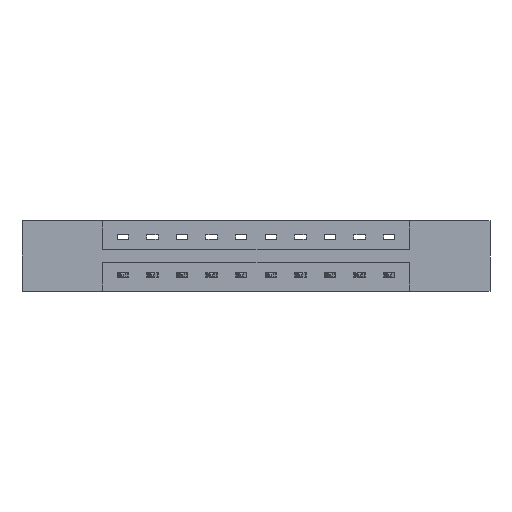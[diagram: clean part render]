
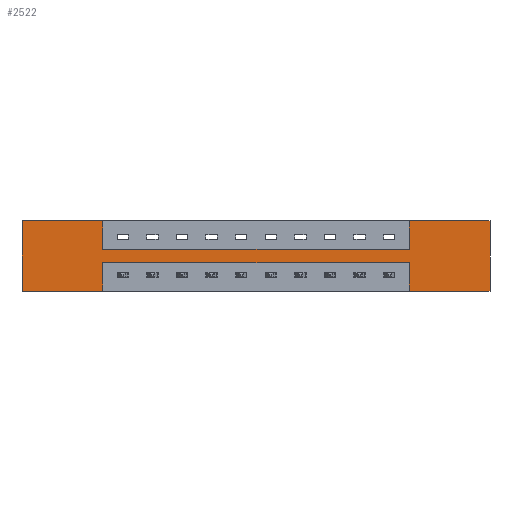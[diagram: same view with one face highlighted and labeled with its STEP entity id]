
A CAD part, front view. The second image highlights one B-rep face of the part: STEP entity #2522.
In plain terms, the highlighted planar face has unit normal (0, -1, 0).
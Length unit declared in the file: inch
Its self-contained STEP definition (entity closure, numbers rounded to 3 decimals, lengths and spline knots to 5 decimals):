
#37 = EDGE_LOOP ( 'NONE', ( #4826, #7178, #9392, #11586, #9649, #265, #9899, #571, #3261, #5677, #7989, #10137 ) ) ;
#176 = LINE ( 'NONE', #4265, #7356 ) ;
#265 = ORIENTED_EDGE ( 'NONE', *, *, #9397, .F. ) ;
#283 = CARTESIAN_POINT ( 'NONE',  ( 2.466, 0., -0.37 ) ) ;
#300 = DIRECTION ( 'NONE',  ( 1., 0., 0. ) ) ;
#311 = VECTOR ( 'NONE', #3619, 39.37008 ) ;
#571 = ORIENTED_EDGE ( 'NONE', *, *, #2666, .F. ) ;
#597 = VECTOR ( 'NONE', #9784, 39.37008 ) ;
#627 = VERTEX_POINT ( 'NONE', #11444 ) ;
#863 = DIRECTION ( 'NONE',  ( 0., -1., 0. ) ) ;
#895 = CARTESIAN_POINT ( 'NONE',  ( 2.041, 0., -0.15 ) ) ;
#914 = CARTESIAN_POINT ( 'NONE',  ( 0., 0., -0.37 ) ) ;
#1224 = VERTEX_POINT ( 'NONE', #1527 ) ;
#1290 = PLANE ( 'NONE',  #4752 ) ;
#1486 = VERTEX_POINT ( 'NONE', #4893 ) ;
#1527 = CARTESIAN_POINT ( 'NONE',  ( 2.466, 0., 0. ) ) ;
#1689 = EDGE_CURVE ( 'NONE', #1224, #8025, #7333, .T. ) ;
#1720 = CARTESIAN_POINT ( 'NONE',  ( 2.041, 0., -0.37 ) ) ;
#1885 = LINE ( 'NONE', #5284, #8769 ) ;
#1949 = EDGE_CURVE ( 'NONE', #8025, #1486, #5438, .T. ) ;
#2281 = CARTESIAN_POINT ( 'NONE',  ( 2.466, 0., 0. ) ) ;
#2320 = DIRECTION ( 'NONE',  ( 0., 0., -1. ) ) ;
#2522 = ADVANCED_FACE ( 'NONE', ( #10419 ), #1290, .T. ) ;
#2524 = DIRECTION ( 'NONE',  ( 0., 0., -1. ) ) ;
#2526 = CARTESIAN_POINT ( 'NONE',  ( 0., 0., -0.37 ) ) ;
#2600 = CARTESIAN_POINT ( 'NONE',  ( 0.425, 0., -0.15 ) ) ;
#2666 = EDGE_CURVE ( 'NONE', #11294, #5237, #2687, .T. ) ;
#2686 = VERTEX_POINT ( 'NONE', #8191 ) ;
#2687 = LINE ( 'NONE', #8328, #6927 ) ;
#2741 = EDGE_CURVE ( 'NONE', #627, #11294, #8667, .T. ) ;
#2843 = CARTESIAN_POINT ( 'NONE',  ( 0., 0., 0. ) ) ;
#3009 = VERTEX_POINT ( 'NONE', #8387 ) ;
#3261 = ORIENTED_EDGE ( 'NONE', *, *, #2741, .F. ) ;
#3354 = VERTEX_POINT ( 'NONE', #7906 ) ;
#3596 = LINE ( 'NONE', #9551, #597 ) ;
#3619 = DIRECTION ( 'NONE',  ( -1., 0., 0. ) ) ;
#4026 = VECTOR ( 'NONE', #9969, 39.37008 ) ;
#4122 = EDGE_CURVE ( 'NONE', #2686, #6451, #8034, .T. ) ;
#4212 = DIRECTION ( 'NONE',  ( -1., 0., 0. ) ) ;
#4265 = CARTESIAN_POINT ( 'NONE',  ( 0., 0., 0. ) ) ;
#4306 = DIRECTION ( 'NONE',  ( 1., 0., 0. ) ) ;
#4416 = EDGE_CURVE ( 'NONE', #3009, #627, #8794, .T. ) ;
#4725 = VECTOR ( 'NONE', #7831, 39.37008 ) ;
#4752 = AXIS2_PLACEMENT_3D ( 'NONE', #914, #863, #2320 ) ;
#4825 = CARTESIAN_POINT ( 'NONE',  ( 0., 0., -0.37 ) ) ;
#4826 = ORIENTED_EDGE ( 'NONE', *, *, #9306, .F. ) ;
#4893 = CARTESIAN_POINT ( 'NONE',  ( 2.041, 0., -0.37 ) ) ;
#4916 = EDGE_CURVE ( 'NONE', #5237, #5583, #3596, .T. ) ;
#5237 = VERTEX_POINT ( 'NONE', #895 ) ;
#5284 = CARTESIAN_POINT ( 'NONE',  ( 0.425, 0., -0.22 ) ) ;
#5314 = EDGE_CURVE ( 'NONE', #11587, #3354, #1885, .T. ) ;
#5438 = LINE ( 'NONE', #4825, #7205 ) ;
#5583 = VERTEX_POINT ( 'NONE', #11512 ) ;
#5677 = ORIENTED_EDGE ( 'NONE', *, *, #4416, .F. ) ;
#6341 = DIRECTION ( 'NONE',  ( 0., 0., 1. ) ) ;
#6451 = VERTEX_POINT ( 'NONE', #9454 ) ;
#6927 = VECTOR ( 'NONE', #4306, 39.37008 ) ;
#6957 = VECTOR ( 'NONE', #2524, 39.37008 ) ;
#7016 = EDGE_CURVE ( 'NONE', #6451, #3009, #10761, .T. ) ;
#7178 = ORIENTED_EDGE ( 'NONE', *, *, #5314, .F. ) ;
#7205 = VECTOR ( 'NONE', #11309, 39.37008 ) ;
#7333 = LINE ( 'NONE', #2281, #9554 ) ;
#7356 = VECTOR ( 'NONE', #300, 39.37008 ) ;
#7831 = DIRECTION ( 'NONE',  ( 1., 0., 0. ) ) ;
#7906 = CARTESIAN_POINT ( 'NONE',  ( 0.425, 0., -0.22 ) ) ;
#7989 = ORIENTED_EDGE ( 'NONE', *, *, #7016, .F. ) ;
#8025 = VERTEX_POINT ( 'NONE', #283 ) ;
#8034 = LINE ( 'NONE', #2526, #311 ) ;
#8191 = CARTESIAN_POINT ( 'NONE',  ( 0.425, 0., -0.37 ) ) ;
#8328 = CARTESIAN_POINT ( 'NONE',  ( 0.425, 0., -0.15 ) ) ;
#8387 = CARTESIAN_POINT ( 'NONE',  ( 0., 0., 0. ) ) ;
#8409 = VECTOR ( 'NONE', #6341, 39.37008 ) ;
#8627 = VECTOR ( 'NONE', #9716, 39.37008 ) ;
#8664 = LINE ( 'NONE', #1720, #8409 ) ;
#8667 = LINE ( 'NONE', #9986, #4026 ) ;
#8769 = VECTOR ( 'NONE', #4212, 39.37008 ) ;
#8794 = LINE ( 'NONE', #10638, #4725 ) ;
#9306 = EDGE_CURVE ( 'NONE', #3354, #2686, #11378, .T. ) ;
#9392 = ORIENTED_EDGE ( 'NONE', *, *, #10572, .F. ) ;
#9397 = EDGE_CURVE ( 'NONE', #5583, #1224, #176, .T. ) ;
#9454 = CARTESIAN_POINT ( 'NONE',  ( 0., 0., -0.37 ) ) ;
#9551 = CARTESIAN_POINT ( 'NONE',  ( 2.041, 0., 0. ) ) ;
#9554 = VECTOR ( 'NONE', #10513, 39.37008 ) ;
#9649 = ORIENTED_EDGE ( 'NONE', *, *, #1689, .F. ) ;
#9716 = DIRECTION ( 'NONE',  ( 0., 0., 1. ) ) ;
#9784 = DIRECTION ( 'NONE',  ( 0., 0., 1. ) ) ;
#9899 = ORIENTED_EDGE ( 'NONE', *, *, #4916, .F. ) ;
#9969 = DIRECTION ( 'NONE',  ( 0., 0., -1. ) ) ;
#9986 = CARTESIAN_POINT ( 'NONE',  ( 0.425, 0., 0. ) ) ;
#10137 = ORIENTED_EDGE ( 'NONE', *, *, #4122, .F. ) ;
#10419 = FACE_OUTER_BOUND ( 'NONE', #37, .T. ) ;
#10513 = DIRECTION ( 'NONE',  ( 0., 0., -1. ) ) ;
#10572 = EDGE_CURVE ( 'NONE', #1486, #11587, #8664, .T. ) ;
#10638 = CARTESIAN_POINT ( 'NONE',  ( 0., 0., 0. ) ) ;
#10761 = LINE ( 'NONE', #2843, #8627 ) ;
#11294 = VERTEX_POINT ( 'NONE', #2600 ) ;
#11309 = DIRECTION ( 'NONE',  ( -1., 0., 0. ) ) ;
#11378 = LINE ( 'NONE', #11385, #6957 ) ;
#11385 = CARTESIAN_POINT ( 'NONE',  ( 0.425, 0., -0.37 ) ) ;
#11444 = CARTESIAN_POINT ( 'NONE',  ( 0.425, 0., 0. ) ) ;
#11512 = CARTESIAN_POINT ( 'NONE',  ( 2.041, 0., 0. ) ) ;
#11552 = CARTESIAN_POINT ( 'NONE',  ( 2.041, 0., -0.22 ) ) ;
#11586 = ORIENTED_EDGE ( 'NONE', *, *, #1949, .F. ) ;
#11587 = VERTEX_POINT ( 'NONE', #11552 ) ;
